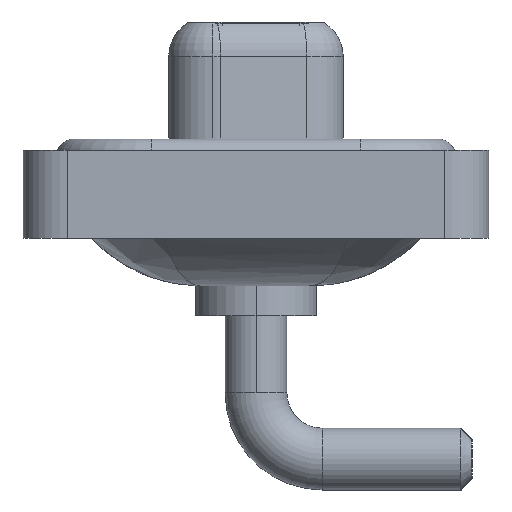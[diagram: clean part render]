
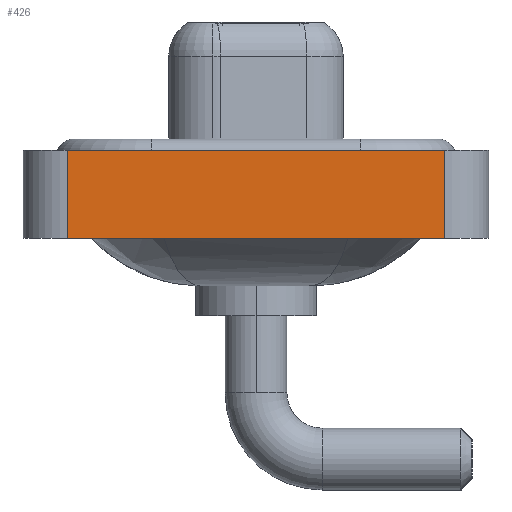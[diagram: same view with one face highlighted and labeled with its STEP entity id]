
A CAD part, left-side view. The second image highlights one B-rep face of the part: STEP entity #426.
In plain terms, the highlighted planar face has unit normal (-1, 0, 0).
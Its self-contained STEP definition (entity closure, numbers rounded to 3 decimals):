
#100 = CARTESIAN_POINT ( 'NONE',  ( -7.25, 8.55, 0.4 ) ) ;
#426 = ADVANCED_FACE ( 'NONE', ( #3863 ), #6614, .T. ) ;
#483 = CARTESIAN_POINT ( 'NONE',  ( -7.25, -8.55, 0.4 ) ) ;
#527 = EDGE_CURVE ( 'NONE', #7364, #15823, #13254, .T. ) ;
#844 = CARTESIAN_POINT ( 'NONE',  ( -7.25, -8.55, -3.6 ) ) ;
#1545 = ORIENTED_EDGE ( 'NONE', *, *, #12213, .T. ) ;
#1957 = LINE ( 'NONE', #10008, #6888 ) ;
#2733 = VECTOR ( 'NONE', #9496, 1000. ) ;
#3001 = CARTESIAN_POINT ( 'NONE',  ( -7.25, 8.55, -3.6 ) ) ;
#3863 = FACE_OUTER_BOUND ( 'NONE', #9254, .T. ) ;
#4246 = DIRECTION ( 'NONE',  ( 0., -1., 0. ) ) ;
#4567 = ORIENTED_EDGE ( 'NONE', *, *, #11340, .F. ) ;
#4700 = DIRECTION ( 'NONE',  ( 0., -1., 0. ) ) ;
#5382 = ORIENTED_EDGE ( 'NONE', *, *, #527, .F. ) ;
#5734 = AXIS2_PLACEMENT_3D ( 'NONE', #11808, #11560, #16783 ) ;
#6535 = VERTEX_POINT ( 'NONE', #13311 ) ;
#6614 = PLANE ( 'NONE',  #5734 ) ;
#6888 = VECTOR ( 'NONE', #7453, 1000. ) ;
#7364 = VERTEX_POINT ( 'NONE', #3001 ) ;
#7453 = DIRECTION ( 'NONE',  ( 0., 0., 1. ) ) ;
#7893 = ORIENTED_EDGE ( 'NONE', *, *, #15432, .T. ) ;
#9254 = EDGE_LOOP ( 'NONE', ( #7893, #4567, #5382, #1545 ) ) ;
#9496 = DIRECTION ( 'NONE',  ( 0., 0., 1. ) ) ;
#10008 = CARTESIAN_POINT ( 'NONE',  ( -7.25, -8.55, -3.6 ) ) ;
#11340 = EDGE_CURVE ( 'NONE', #15823, #6535, #13547, .T. ) ;
#11560 = DIRECTION ( 'NONE',  ( -1., 0., 0. ) ) ;
#11808 = CARTESIAN_POINT ( 'NONE',  ( -7.25, -8.55, -3.6 ) ) ;
#12213 = EDGE_CURVE ( 'NONE', #7364, #14712, #15931, .T. ) ;
#13179 = VECTOR ( 'NONE', #4700, 1000. ) ;
#13254 = LINE ( 'NONE', #13418, #2733 ) ;
#13311 = CARTESIAN_POINT ( 'NONE',  ( -7.25, -8.55, 0.4 ) ) ;
#13418 = CARTESIAN_POINT ( 'NONE',  ( -7.25, 8.55, -3.6 ) ) ;
#13547 = LINE ( 'NONE', #483, #15958 ) ;
#13871 = CARTESIAN_POINT ( 'NONE',  ( -7.25, -8.55, -3.6 ) ) ;
#14712 = VERTEX_POINT ( 'NONE', #13871 ) ;
#15432 = EDGE_CURVE ( 'NONE', #14712, #6535, #1957, .T. ) ;
#15823 = VERTEX_POINT ( 'NONE', #100 ) ;
#15931 = LINE ( 'NONE', #844, #13179 ) ;
#15958 = VECTOR ( 'NONE', #4246, 1000. ) ;
#16783 = DIRECTION ( 'NONE',  ( 0., 0., 1. ) ) ;
